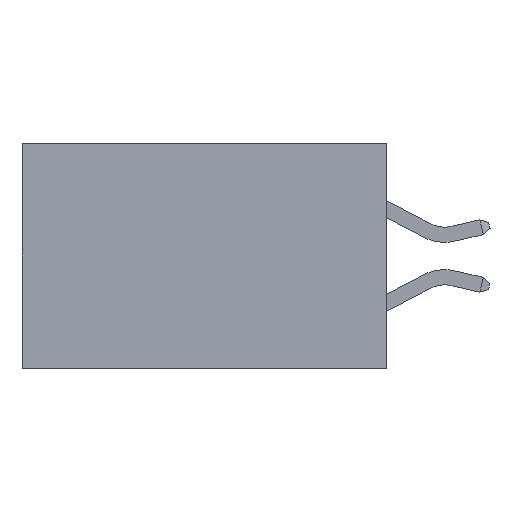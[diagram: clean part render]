
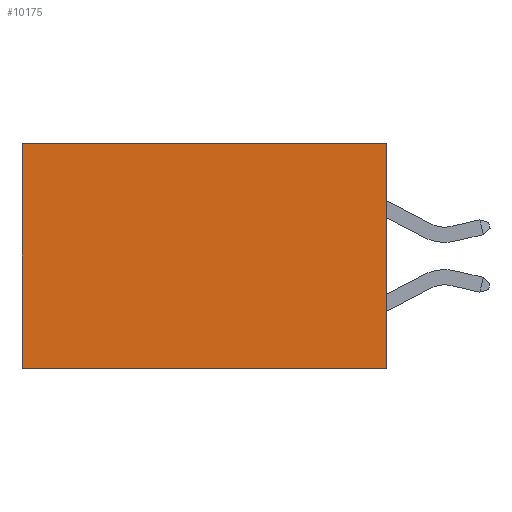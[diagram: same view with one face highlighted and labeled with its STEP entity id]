
A CAD part, left-side view. The second image highlights one B-rep face of the part: STEP entity #10175.
In plain terms, the highlighted planar face has unit normal (-1, 0, 0).
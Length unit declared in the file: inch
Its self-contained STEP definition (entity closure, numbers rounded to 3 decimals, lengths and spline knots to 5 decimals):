
#394 = CARTESIAN_POINT ( 'NONE',  ( 0.298, 0.6, 0. ) ) ;
#1101 = ORIENTED_EDGE ( 'NONE', *, *, #7233, .F. ) ;
#1112 = ORIENTED_EDGE ( 'NONE', *, *, #5465, .T. ) ;
#1827 = CARTESIAN_POINT ( 'NONE',  ( 0.298, 0., -0.37 ) ) ;
#2163 = VECTOR ( 'NONE', #6038, 39.37008 ) ;
#2224 = DIRECTION ( 'NONE',  ( 0., 1., 0. ) ) ;
#2238 = VERTEX_POINT ( 'NONE', #2923 ) ;
#2349 = CARTESIAN_POINT ( 'NONE',  ( 0.298, 0.6, -0.37 ) ) ;
#2418 = LINE ( 'NONE', #9158, #2163 ) ;
#2777 = PLANE ( 'NONE',  #10311 ) ;
#2815 = DIRECTION ( 'NONE',  ( 1., 0., 0. ) ) ;
#2861 = CARTESIAN_POINT ( 'NONE',  ( 0.298, 0.6, 0. ) ) ;
#2923 = CARTESIAN_POINT ( 'NONE',  ( 0.298, 0., 0. ) ) ;
#3571 = DIRECTION ( 'NONE',  ( 0., 0., -1. ) ) ;
#4135 = FACE_OUTER_BOUND ( 'NONE', #8603, .T. ) ;
#4664 = VECTOR ( 'NONE', #3571, 39.37008 ) ;
#4793 = LINE ( 'NONE', #7225, #4942 ) ;
#4942 = VECTOR ( 'NONE', #5794, 39.37008 ) ;
#5397 = ORIENTED_EDGE ( 'NONE', *, *, #5687, .F. ) ;
#5465 = EDGE_CURVE ( 'NONE', #8831, #9070, #10468, .T. ) ;
#5687 = EDGE_CURVE ( 'NONE', #2238, #7292, #4793, .T. ) ;
#5757 = ORIENTED_EDGE ( 'NONE', *, *, #5898, .T. ) ;
#5794 = DIRECTION ( 'NONE',  ( 0., 0., -1. ) ) ;
#5898 = EDGE_CURVE ( 'NONE', #2238, #8831, #2418, .T. ) ;
#6038 = DIRECTION ( 'NONE',  ( 0., 1., 0. ) ) ;
#7225 = CARTESIAN_POINT ( 'NONE',  ( 0.298, 0., 0. ) ) ;
#7233 = EDGE_CURVE ( 'NONE', #7292, #9070, #8955, .T. ) ;
#7292 = VERTEX_POINT ( 'NONE', #1827 ) ;
#7854 = CARTESIAN_POINT ( 'NONE',  ( 0.298, 0., 0. ) ) ;
#8603 = EDGE_LOOP ( 'NONE', ( #1112, #1101, #5397, #5757 ) ) ;
#8607 = DIRECTION ( 'NONE',  ( 0., 0., -1. ) ) ;
#8831 = VERTEX_POINT ( 'NONE', #394 ) ;
#8955 = LINE ( 'NONE', #9515, #9174 ) ;
#9070 = VERTEX_POINT ( 'NONE', #2349 ) ;
#9158 = CARTESIAN_POINT ( 'NONE',  ( 0.298, 0., 0. ) ) ;
#9174 = VECTOR ( 'NONE', #2224, 39.37008 ) ;
#9515 = CARTESIAN_POINT ( 'NONE',  ( 0.298, 0., -0.37 ) ) ;
#10175 = ADVANCED_FACE ( 'NONE', ( #4135 ), #2777, .F. ) ;
#10311 = AXIS2_PLACEMENT_3D ( 'NONE', #7854, #2815, #8607 ) ;
#10468 = LINE ( 'NONE', #2861, #4664 ) ;
